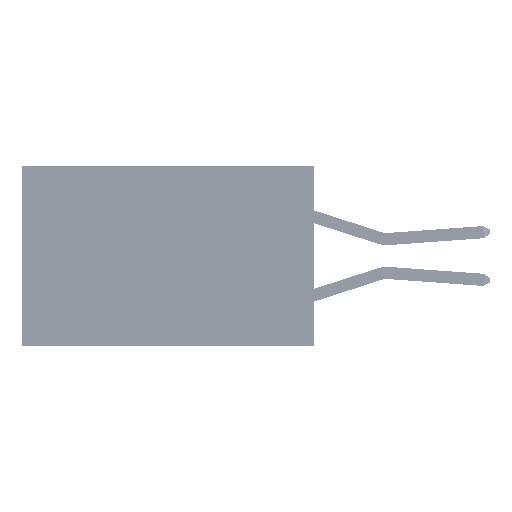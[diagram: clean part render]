
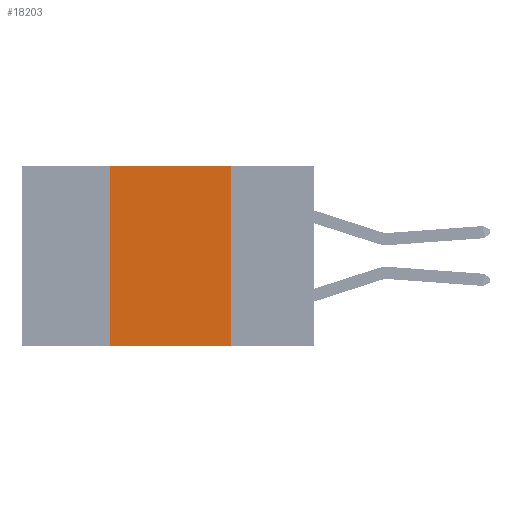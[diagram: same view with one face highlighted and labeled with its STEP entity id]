
A CAD part, left-side view. The second image highlights one B-rep face of the part: STEP entity #18203.
In plain terms, the highlighted planar face has unit normal (-1, 0, 0).
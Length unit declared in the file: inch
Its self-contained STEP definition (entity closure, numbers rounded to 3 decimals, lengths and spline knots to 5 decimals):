
#1049 = CARTESIAN_POINT ( 'NONE',  ( 0., 0.6, 0. ) ) ;
#5187 = VERTEX_POINT ( 'NONE', #46201 ) ;
#7587 = LINE ( 'NONE', #21265, #38397 ) ;
#8464 = ORIENTED_EDGE ( 'NONE', *, *, #26455, .F. ) ;
#10263 = EDGE_CURVE ( 'NONE', #11902, #43281, #34916, .T. ) ;
#10412 = AXIS2_PLACEMENT_3D ( 'NONE', #1049, #17167, #45292 ) ;
#10918 = VERTEX_POINT ( 'NONE', #17867 ) ;
#11630 = CARTESIAN_POINT ( 'NONE',  ( 0., 0.42, -0.37 ) ) ;
#11902 = VERTEX_POINT ( 'NONE', #11630 ) ;
#14930 = CARTESIAN_POINT ( 'NONE',  ( 0., 0.6, 0. ) ) ;
#14993 = FACE_OUTER_BOUND ( 'NONE', #39169, .T. ) ;
#16871 = ORIENTED_EDGE ( 'NONE', *, *, #10263, .F. ) ;
#17167 = DIRECTION ( 'NONE',  ( 1., 0., 0. ) ) ;
#17867 = CARTESIAN_POINT ( 'NONE',  ( 0., 0.17, -0.37 ) ) ;
#18203 = ADVANCED_FACE ( 'NONE', ( #14993 ), #41288, .F. ) ;
#21084 = ORIENTED_EDGE ( 'NONE', *, *, #28193, .F. ) ;
#21265 = CARTESIAN_POINT ( 'NONE',  ( 0., 0.17, 0. ) ) ;
#24130 = ORIENTED_EDGE ( 'NONE', *, *, #46955, .T. ) ;
#24886 = CARTESIAN_POINT ( 'NONE',  ( 0., 0.42, 0. ) ) ;
#25331 = DIRECTION ( 'NONE',  ( 0., 0., -1. ) ) ;
#25475 = VECTOR ( 'NONE', #37840, 39.37008 ) ;
#26455 = EDGE_CURVE ( 'NONE', #5187, #10918, #7587, .T. ) ;
#27537 = CARTESIAN_POINT ( 'NONE',  ( 0., 0.6, -0.37 ) ) ;
#28193 = EDGE_CURVE ( 'NONE', #43281, #5187, #33861, .T. ) ;
#32800 = VECTOR ( 'NONE', #43635, 39.37008 ) ;
#33831 = CARTESIAN_POINT ( 'NONE',  ( 0., 0.42, 0. ) ) ;
#33861 = LINE ( 'NONE', #14930, #43230 ) ;
#34058 = LINE ( 'NONE', #27537, #32800 ) ;
#34916 = LINE ( 'NONE', #33831, #25475 ) ;
#37840 = DIRECTION ( 'NONE',  ( 0., 0., 1. ) ) ;
#38397 = VECTOR ( 'NONE', #25331, 39.37008 ) ;
#39040 = DIRECTION ( 'NONE',  ( 0., -1., 0. ) ) ;
#39169 = EDGE_LOOP ( 'NONE', ( #8464, #21084, #16871, #24130 ) ) ;
#41288 = PLANE ( 'NONE',  #10412 ) ;
#43230 = VECTOR ( 'NONE', #39040, 39.37008 ) ;
#43281 = VERTEX_POINT ( 'NONE', #24886 ) ;
#43635 = DIRECTION ( 'NONE',  ( 0., -1., 0. ) ) ;
#45292 = DIRECTION ( 'NONE',  ( 0., 0., -1. ) ) ;
#46201 = CARTESIAN_POINT ( 'NONE',  ( 0., 0.17, 0. ) ) ;
#46955 = EDGE_CURVE ( 'NONE', #11902, #10918, #34058, .T. ) ;
